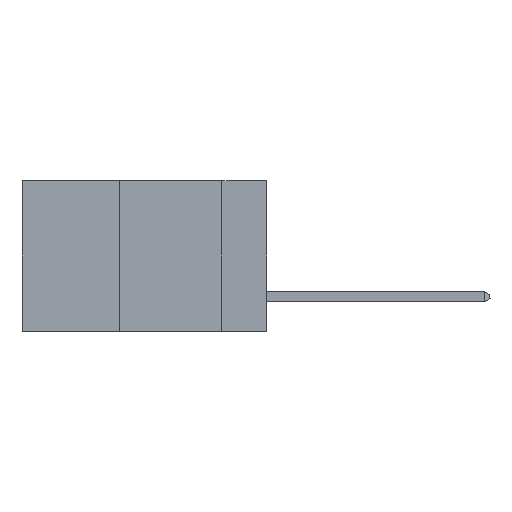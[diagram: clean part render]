
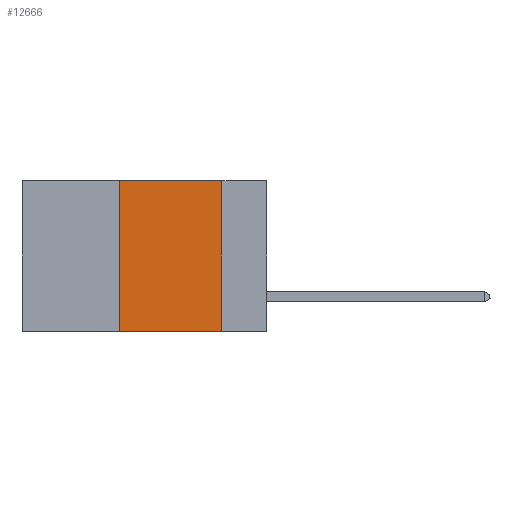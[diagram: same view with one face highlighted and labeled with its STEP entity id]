
A CAD part, left-side view. The second image highlights one B-rep face of the part: STEP entity #12666.
In plain terms, the highlighted planar face has unit normal (-1, 0, 0).
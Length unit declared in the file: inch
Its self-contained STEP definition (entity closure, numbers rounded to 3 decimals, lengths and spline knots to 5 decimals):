
#101 = CARTESIAN_POINT ( 'NONE',  ( 0., 0.6, 0. ) ) ;
#407 = CARTESIAN_POINT ( 'NONE',  ( 0., 0.36, 0. ) ) ;
#2309 = CARTESIAN_POINT ( 'NONE',  ( 0., 0.6, -0.37 ) ) ;
#2455 = EDGE_CURVE ( 'NONE', #8122, #4432, #6726, .T. ) ;
#3195 = ORIENTED_EDGE ( 'NONE', *, *, #10119, .F. ) ;
#3910 = DIRECTION ( 'NONE',  ( 1., 0., 0. ) ) ;
#4274 = CARTESIAN_POINT ( 'NONE',  ( 0., 0.11, -0.37 ) ) ;
#4432 = VERTEX_POINT ( 'NONE', #4274 ) ;
#5446 = PLANE ( 'NONE',  #14467 ) ;
#5794 = CARTESIAN_POINT ( 'NONE',  ( 0., 0.6, 0. ) ) ;
#6726 = LINE ( 'NONE', #2309, #13185 ) ;
#7435 = VECTOR ( 'NONE', #14338, 39.37008 ) ;
#7814 = CARTESIAN_POINT ( 'NONE',  ( 0., 0.11, 0. ) ) ;
#8122 = VERTEX_POINT ( 'NONE', #11103 ) ;
#8258 = CARTESIAN_POINT ( 'NONE',  ( 0., 0.36, 0. ) ) ;
#8730 = EDGE_CURVE ( 'NONE', #8122, #10550, #9125, .T. ) ;
#9031 = DIRECTION ( 'NONE',  ( 0., -1., 0. ) ) ;
#9125 = LINE ( 'NONE', #8258, #14400 ) ;
#9174 = VERTEX_POINT ( 'NONE', #10131 ) ;
#9473 = DIRECTION ( 'NONE',  ( 0., -1., 0. ) ) ;
#9728 = EDGE_CURVE ( 'NONE', #10550, #9174, #13735, .T. ) ;
#10119 = EDGE_CURVE ( 'NONE', #9174, #4432, #15802, .T. ) ;
#10131 = CARTESIAN_POINT ( 'NONE',  ( 0., 0.11, 0. ) ) ;
#10525 = VECTOR ( 'NONE', #9473, 39.37008 ) ;
#10550 = VERTEX_POINT ( 'NONE', #407 ) ;
#10836 = ORIENTED_EDGE ( 'NONE', *, *, #8730, .F. ) ;
#11103 = CARTESIAN_POINT ( 'NONE',  ( 0., 0.36, -0.37 ) ) ;
#11713 = DIRECTION ( 'NONE',  ( 0., 0., -1. ) ) ;
#11812 = FACE_OUTER_BOUND ( 'NONE', #14056, .T. ) ;
#12529 = ORIENTED_EDGE ( 'NONE', *, *, #2455, .T. ) ;
#12666 = ADVANCED_FACE ( 'NONE', ( #11812 ), #5446, .F. ) ;
#13059 = ORIENTED_EDGE ( 'NONE', *, *, #9728, .F. ) ;
#13185 = VECTOR ( 'NONE', #9031, 39.37008 ) ;
#13735 = LINE ( 'NONE', #5794, #10525 ) ;
#14056 = EDGE_LOOP ( 'NONE', ( #3195, #13059, #10836, #12529 ) ) ;
#14338 = DIRECTION ( 'NONE',  ( 0., 0., -1. ) ) ;
#14400 = VECTOR ( 'NONE', #14799, 39.37008 ) ;
#14467 = AXIS2_PLACEMENT_3D ( 'NONE', #101, #3910, #11713 ) ;
#14799 = DIRECTION ( 'NONE',  ( 0., 0., 1. ) ) ;
#15802 = LINE ( 'NONE', #7814, #7435 ) ;
